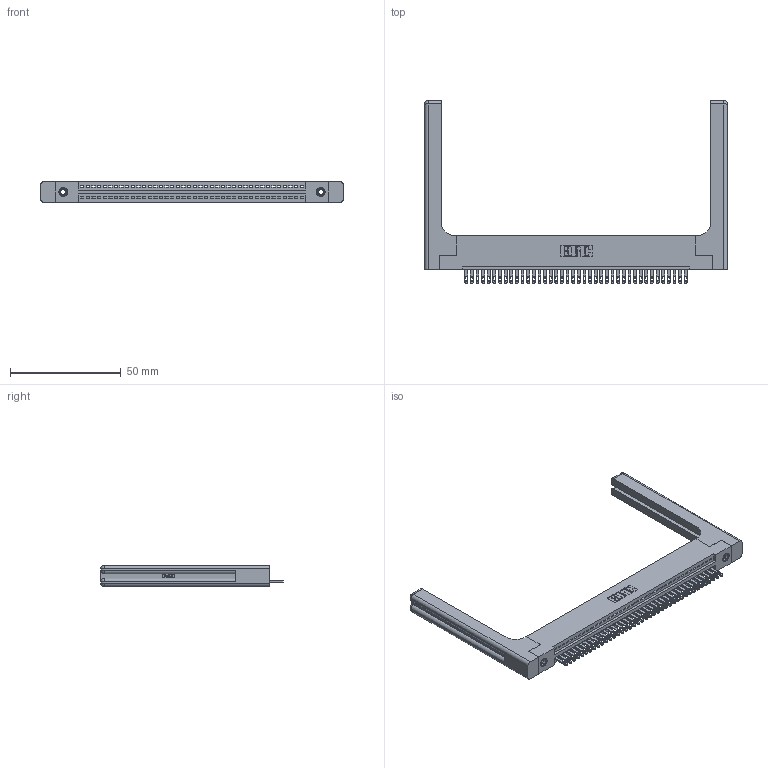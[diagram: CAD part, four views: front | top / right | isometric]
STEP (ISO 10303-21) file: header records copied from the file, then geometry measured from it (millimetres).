
FILE_DESCRIPTION (( 'STEP AP203' ), '1' );
FILE_NAME ('345-040-500-158.STEP', '2019-10-08T07:56:56', ( '' ), ( '' ), 'SwSTEP 2.0', 'SolidWorks 2016', '' );
FILE_SCHEMA (( 'CONFIG_CONTROL_DESIGN' ));
Length unit declared in the file: inch
Products named in the file (5): 345-292-001_345-293-100; 345-250-001_345-250-001-102; 345 Part_Flush Mounting Lugs - 0.156 Dia-TH; 345-220-058_345-220-058; 345-040-500-158
Assembly tree (45 placements, depth 2):
  345-040-500-158
    345 Part_Flush Mounting Lugs - 0.156 Dia-TH
    345-292-001_345-293-100  x40
    345-250-001_345-250-001-102  x2
    345-220-058_345-220-058  x2
Bounding box: 136.63 x 82.47 x 9.4 mm (x, y, z)
Volume: 21490.3 mm3; surface area: 22624.5 mm2
Topology: 45 solids, 45 shells, 2542 faces, 7727 edges, 5130 vertices
Faces by surface type: plane 1588, cylinder 894, bspline 36, cone 12, sphere 8, torus 4
Entity records: 35486 total; most frequent: CARTESIAN_POINT 7117, ORIENTED_EDGE 5888, DIRECTION 5168, EDGE_CURVE 2944, LINE 2556, VECTOR 2556, VERTEX_POINT 1954, AXIS2_PLACEMENT_3D 1306
